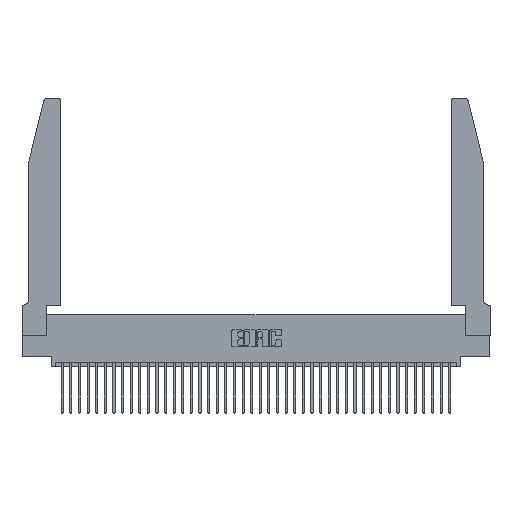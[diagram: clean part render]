
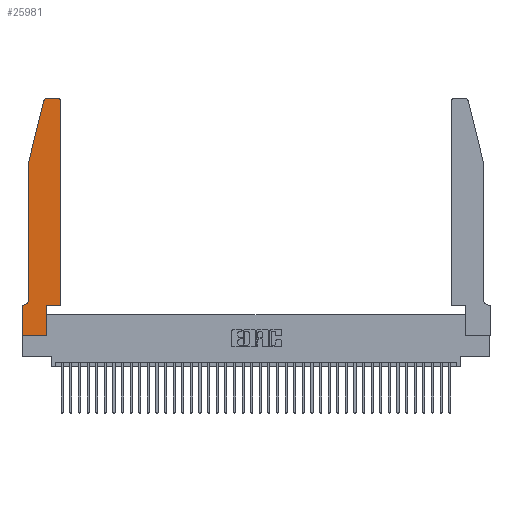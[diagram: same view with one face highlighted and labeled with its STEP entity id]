
A CAD part, top view. The second image highlights one B-rep face of the part: STEP entity #25981.
In plain terms, the highlighted planar face has unit normal (0, 0, 1).
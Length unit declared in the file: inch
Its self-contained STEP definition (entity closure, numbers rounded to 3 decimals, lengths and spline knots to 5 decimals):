
#296 = VECTOR ( 'NONE', #23118, 39.37008 ) ;
#349 = CARTESIAN_POINT ( 'NONE',  ( 0.0055, 0.35, 0.37 ) ) ;
#1424 = ORIENTED_EDGE ( 'NONE', *, *, #31346, .T. ) ;
#1440 = EDGE_CURVE ( 'NONE', #20427, #26528, #20175, .T. ) ;
#1647 = VECTOR ( 'NONE', #27409, 39.37008 ) ;
#1893 = DIRECTION ( 'NONE',  ( 0., 0., 1. ) ) ;
#2781 = ORIENTED_EDGE ( 'NONE', *, *, #33763, .T. ) ;
#3001 = DIRECTION ( 'NONE',  ( -1., 0., 0. ) ) ;
#3193 = VERTEX_POINT ( 'NONE', #17461 ) ;
#3936 = CARTESIAN_POINT ( 'NONE',  ( 0.2865, 0.35, 0.37 ) ) ;
#4601 = ORIENTED_EDGE ( 'NONE', *, *, #26518, .T. ) ;
#5017 = ORIENTED_EDGE ( 'NONE', *, *, #39388, .T. ) ;
#5444 = CIRCLE ( 'NONE', #21357, 0.03 ) ;
#5474 = ORIENTED_EDGE ( 'NONE', *, *, #1440, .T. ) ;
#5643 = LINE ( 'NONE', #13663, #30671 ) ;
#6375 = CARTESIAN_POINT ( 'NONE',  ( 0.4505, 0.35, 0.37 ) ) ;
#6598 = ORIENTED_EDGE ( 'NONE', *, *, #36774, .T. ) ;
#6963 = CARTESIAN_POINT ( 'NONE',  ( 0.2865, 0.35, 0.37 ) ) ;
#7174 = ORIENTED_EDGE ( 'NONE', *, *, #35958, .T. ) ;
#8270 = DIRECTION ( 'NONE',  ( 0., -1., 0. ) ) ;
#8817 = LINE ( 'NONE', #22978, #296 ) ;
#8826 = DIRECTION ( 'NONE',  ( 1., 0., 0. ) ) ;
#9060 = ORIENTED_EDGE ( 'NONE', *, *, #18921, .T. ) ;
#9325 = CARTESIAN_POINT ( 'NONE',  ( 0., 0.35, 0.37 ) ) ;
#9328 = VECTOR ( 'NONE', #29974, 39.37008 ) ;
#9931 = CARTESIAN_POINT ( 'NONE',  ( 0., 0., 0.37 ) ) ;
#10150 = LINE ( 'NONE', #24273, #1647 ) ;
#10156 = DIRECTION ( 'NONE',  ( 0., 1., 0. ) ) ;
#11266 = CARTESIAN_POINT ( 'NONE',  ( 0.2605, 2.75, 0.37 ) ) ;
#12559 = DIRECTION ( 'NONE',  ( 0., 0., 1. ) ) ;
#12560 = CARTESIAN_POINT ( 'NONE',  ( 0.4505, 2.72, 0.37 ) ) ;
#12680 = VECTOR ( 'NONE', #8826, 39.37008 ) ;
#13057 = ORIENTED_EDGE ( 'NONE', *, *, #24478, .T. ) ;
#13663 = CARTESIAN_POINT ( 'NONE',  ( 0.0755, 0.35, 0.37 ) ) ;
#13978 = LINE ( 'NONE', #6963, #27604 ) ;
#14222 = ORIENTED_EDGE ( 'NONE', *, *, #23002, .T. ) ;
#14229 = VERTEX_POINT ( 'NONE', #6375 ) ;
#14532 = CARTESIAN_POINT ( 'NONE',  ( 0.25487, 2.72718, 0.37 ) ) ;
#15060 = CARTESIAN_POINT ( 'NONE',  ( 0.284, 2.72, 0.37 ) ) ;
#15303 = AXIS2_PLACEMENT_3D ( 'NONE', #15060, #36657, #18224 ) ;
#15911 = DIRECTION ( 'NONE',  ( 0., 1., 0. ) ) ;
#16382 = VERTEX_POINT ( 'NONE', #12560 ) ;
#16630 = EDGE_CURVE ( 'NONE', #19454, #33935, #5643, .T. ) ;
#17316 = VERTEX_POINT ( 'NONE', #3936 ) ;
#17461 = CARTESIAN_POINT ( 'NONE',  ( 0.4205, 2.75, 0.37 ) ) ;
#17598 = CARTESIAN_POINT ( 'NONE',  ( 0.0755, 2., 0.37 ) ) ;
#17888 = CARTESIAN_POINT ( 'NONE',  ( 0., 0., 0.37 ) ) ;
#17890 = CIRCLE ( 'NONE', #15303, 0.03 ) ;
#18224 = DIRECTION ( 'NONE',  ( 1., 0., 0. ) ) ;
#18290 = CARTESIAN_POINT ( 'NONE',  ( 0.4505, 0.35, 0.37 ) ) ;
#18417 = VERTEX_POINT ( 'NONE', #18625 ) ;
#18625 = CARTESIAN_POINT ( 'NONE',  ( 0.2865, 0., 0.37 ) ) ;
#18921 = EDGE_CURVE ( 'NONE', #16382, #3193, #5444, .T. ) ;
#19352 = CARTESIAN_POINT ( 'NONE',  ( 0.284, 2.75, 0.37 ) ) ;
#19454 = VERTEX_POINT ( 'NONE', #349 ) ;
#19764 = LINE ( 'NONE', #37485, #37069 ) ;
#20175 = LINE ( 'NONE', #38830, #34630 ) ;
#20427 = VERTEX_POINT ( 'NONE', #17598 ) ;
#20919 = CARTESIAN_POINT ( 'NONE',  ( 0.4205, 2.72, 0.37 ) ) ;
#21357 = AXIS2_PLACEMENT_3D ( 'NONE', #20919, #1893, #23996 ) ;
#22000 = DIRECTION ( 'NONE',  ( 0., 0., -1. ) ) ;
#22303 = LINE ( 'NONE', #17888, #30526 ) ;
#22978 = CARTESIAN_POINT ( 'NONE',  ( 0.0755, 2., 0.37 ) ) ;
#23002 = EDGE_CURVE ( 'NONE', #18417, #17316, #13978, .T. ) ;
#23118 = DIRECTION ( 'NONE',  ( -0.239, -0.971, 0. ) ) ;
#23996 = DIRECTION ( 'NONE',  ( 1., 0., 0. ) ) ;
#24273 = CARTESIAN_POINT ( 'NONE',  ( 0., 0., 0.37 ) ) ;
#24478 = EDGE_CURVE ( 'NONE', #24662, #20427, #8817, .T. ) ;
#24662 = VERTEX_POINT ( 'NONE', #14532 ) ;
#25981 = ADVANCED_FACE ( 'NONE', ( #29761 ), #28115, .T. ) ;
#26518 = EDGE_CURVE ( 'NONE', #37789, #18417, #10150, .T. ) ;
#26528 = VERTEX_POINT ( 'NONE', #30499 ) ;
#26678 = DIRECTION ( 'NONE',  ( 0., -1., 0. ) ) ;
#27028 = LINE ( 'NONE', #11266, #9328 ) ;
#27409 = DIRECTION ( 'NONE',  ( 1., 0., 0. ) ) ;
#27604 = VECTOR ( 'NONE', #10156, 39.37008 ) ;
#28115 = PLANE ( 'NONE',  #40247 ) ;
#29761 = FACE_OUTER_BOUND ( 'NONE', #32053, .T. ) ;
#29974 = DIRECTION ( 'NONE',  ( -1., 0., 0. ) ) ;
#30499 = CARTESIAN_POINT ( 'NONE',  ( 0.0755, 0.42, 0.37 ) ) ;
#30526 = VECTOR ( 'NONE', #8270, 39.37008 ) ;
#30671 = VECTOR ( 'NONE', #32273, 39.37008 ) ;
#30861 = VERTEX_POINT ( 'NONE', #19352 ) ;
#31346 = EDGE_CURVE ( 'NONE', #26528, #19454, #34454, .T. ) ;
#31537 = ORIENTED_EDGE ( 'NONE', *, *, #32365, .T. ) ;
#31811 = AXIS2_PLACEMENT_3D ( 'NONE', #40374, #22000, #3001 ) ;
#32053 = EDGE_LOOP ( 'NONE', ( #6598, #7174, #13057, #5474, #1424, #33385, #31537, #4601, #14222, #5017, #2781, #9060 ) ) ;
#32273 = DIRECTION ( 'NONE',  ( -1., 0., 0. ) ) ;
#32365 = EDGE_CURVE ( 'NONE', #33935, #37789, #22303, .T. ) ;
#33385 = ORIENTED_EDGE ( 'NONE', *, *, #16630, .T. ) ;
#33763 = EDGE_CURVE ( 'NONE', #14229, #16382, #19764, .T. ) ;
#33935 = VERTEX_POINT ( 'NONE', #38264 ) ;
#34300 = DIRECTION ( 'NONE',  ( 1., 0., 0. ) ) ;
#34454 = CIRCLE ( 'NONE', #31811, 0.07 ) ;
#34630 = VECTOR ( 'NONE', #26678, 39.37008 ) ;
#35958 = EDGE_CURVE ( 'NONE', #30861, #24662, #17890, .T. ) ;
#36657 = DIRECTION ( 'NONE',  ( 0., 0., 1. ) ) ;
#36774 = EDGE_CURVE ( 'NONE', #3193, #30861, #27028, .T. ) ;
#37069 = VECTOR ( 'NONE', #15911, 39.37008 ) ;
#37485 = CARTESIAN_POINT ( 'NONE',  ( 0.4505, 0.35, 0.37 ) ) ;
#37789 = VERTEX_POINT ( 'NONE', #9931 ) ;
#38264 = CARTESIAN_POINT ( 'NONE',  ( 0., 0.35, 0.37 ) ) ;
#38343 = LINE ( 'NONE', #18290, #12680 ) ;
#38830 = CARTESIAN_POINT ( 'NONE',  ( 0.0755, 2., 0.37 ) ) ;
#39388 = EDGE_CURVE ( 'NONE', #17316, #14229, #38343, .T. ) ;
#40247 = AXIS2_PLACEMENT_3D ( 'NONE', #9325, #12559, #34300 ) ;
#40374 = CARTESIAN_POINT ( 'NONE',  ( 0.0055, 0.42, 0.37 ) ) ;
